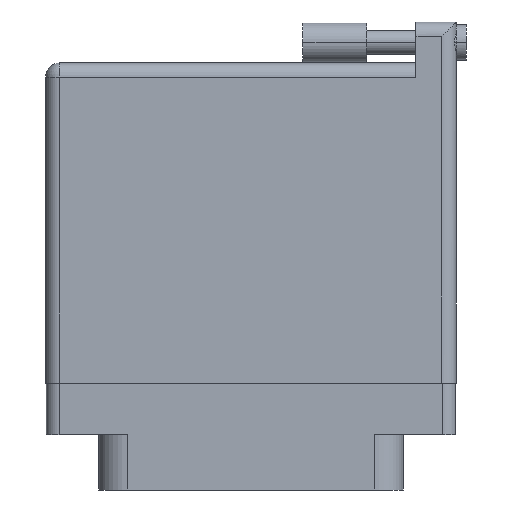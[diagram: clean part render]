
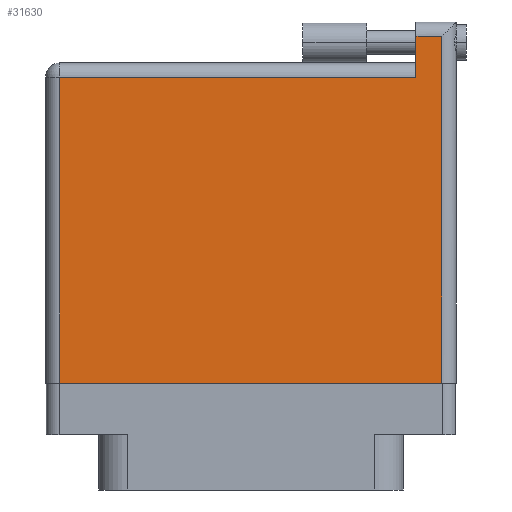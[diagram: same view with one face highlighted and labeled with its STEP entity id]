
A CAD part, front view. The second image highlights one B-rep face of the part: STEP entity #31630.
In plain terms, the highlighted face is planar.
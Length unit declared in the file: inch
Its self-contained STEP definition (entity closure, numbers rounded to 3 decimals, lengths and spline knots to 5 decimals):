
#173 = CARTESIAN_POINT ( 'NONE',  ( -0.934, 1.396, 0.4495 ) ) ;
#1658 = VECTOR ( 'NONE', #15716, 39.37008 ) ;
#1914 = VECTOR ( 'NONE', #25985, 39.37008 ) ;
#2042 = CARTESIAN_POINT ( 'NONE',  ( 0.934, 1.596, 0.4495 ) ) ;
#2191 = CARTESIAN_POINT ( 'NONE',  ( -1.004, 1.396, 0.4495 ) ) ;
#2243 = CARTESIAN_POINT ( 'NONE',  ( 0.807, 1.396, 0.4495 ) ) ;
#5108 = EDGE_LOOP ( 'NONE', ( #27374, #22865, #27792, #35774, #8411, #16179 ) ) ;
#6173 = EDGE_CURVE ( 'NONE', #32402, #24748, #17242, .T. ) ;
#6331 = VECTOR ( 'NONE', #27224, 39.37008 ) ;
#7797 = EDGE_CURVE ( 'NONE', #24748, #8620, #35243, .T. ) ;
#8411 = ORIENTED_EDGE ( 'NONE', *, *, #19069, .T. ) ;
#8620 = VERTEX_POINT ( 'NONE', #2042 ) ;
#8821 = CARTESIAN_POINT ( 'NONE',  ( -0.934, -0.1, 0.4495 ) ) ;
#9067 = DIRECTION ( 'NONE',  ( 0., -1., 0. ) ) ;
#9209 = EDGE_CURVE ( 'NONE', #20567, #34729, #27019, .T. ) ;
#9238 = CARTESIAN_POINT ( 'NONE',  ( -1.004, 1.596, 0.4495 ) ) ;
#9274 = FACE_OUTER_BOUND ( 'NONE', #5108, .T. ) ;
#9311 = CARTESIAN_POINT ( 'NONE',  ( -0.934, -0.1, 0.4495 ) ) ;
#9957 = VECTOR ( 'NONE', #13397, 39.37008 ) ;
#10689 = VECTOR ( 'NONE', #23078, 39.37008 ) ;
#11922 = EDGE_CURVE ( 'NONE', #18264, #32402, #27705, .T. ) ;
#13397 = DIRECTION ( 'NONE',  ( -1., 0., 0. ) ) ;
#13559 = CARTESIAN_POINT ( 'NONE',  ( 0.934, 1.666, 0.4495 ) ) ;
#15640 = VECTOR ( 'NONE', #9067, 39.37008 ) ;
#15716 = DIRECTION ( 'NONE',  ( 1., 0., 0. ) ) ;
#15832 = CARTESIAN_POINT ( 'NONE',  ( -1.004, -0.1, 0.4495 ) ) ;
#16024 = DIRECTION ( 'NONE',  ( -1., 0., 0. ) ) ;
#16179 = ORIENTED_EDGE ( 'NONE', *, *, #11922, .T. ) ;
#17242 = LINE ( 'NONE', #15832, #1658 ) ;
#17755 = CARTESIAN_POINT ( 'NONE',  ( 0.807, 1.666, 0.4495 ) ) ;
#18264 = VERTEX_POINT ( 'NONE', #173 ) ;
#19053 = PLANE ( 'NONE',  #25565 ) ;
#19069 = EDGE_CURVE ( 'NONE', #34729, #18264, #22589, .T. ) ;
#20567 = VERTEX_POINT ( 'NONE', #31890 ) ;
#21007 = EDGE_CURVE ( 'NONE', #8620, #20567, #27565, .T. ) ;
#22056 = DIRECTION ( 'NONE',  ( 0., 0., -1. ) ) ;
#22589 = LINE ( 'NONE', #2191, #9957 ) ;
#22865 = ORIENTED_EDGE ( 'NONE', *, *, #7797, .T. ) ;
#23078 = DIRECTION ( 'NONE',  ( -1., 0., 0. ) ) ;
#24748 = VERTEX_POINT ( 'NONE', #30724 ) ;
#25565 = AXIS2_PLACEMENT_3D ( 'NONE', #32893, #22056, #16024 ) ;
#25985 = DIRECTION ( 'NONE',  ( 0., -1., 0. ) ) ;
#27019 = LINE ( 'NONE', #17755, #1914 ) ;
#27224 = DIRECTION ( 'NONE',  ( 0., 1., 0. ) ) ;
#27374 = ORIENTED_EDGE ( 'NONE', *, *, #6173, .T. ) ;
#27565 = LINE ( 'NONE', #9238, #10689 ) ;
#27705 = LINE ( 'NONE', #9311, #15640 ) ;
#27792 = ORIENTED_EDGE ( 'NONE', *, *, #21007, .T. ) ;
#30724 = CARTESIAN_POINT ( 'NONE',  ( 0.934, -0.1, 0.4495 ) ) ;
#31630 = ADVANCED_FACE ( 'NONE', ( #9274 ), #19053, .F. ) ;
#31890 = CARTESIAN_POINT ( 'NONE',  ( 0.807, 1.596, 0.4495 ) ) ;
#32402 = VERTEX_POINT ( 'NONE', #8821 ) ;
#32893 = CARTESIAN_POINT ( 'NONE',  ( -1.004, 1.466, 0.4495 ) ) ;
#34729 = VERTEX_POINT ( 'NONE', #2243 ) ;
#35243 = LINE ( 'NONE', #13559, #6331 ) ;
#35774 = ORIENTED_EDGE ( 'NONE', *, *, #9209, .T. ) ;
